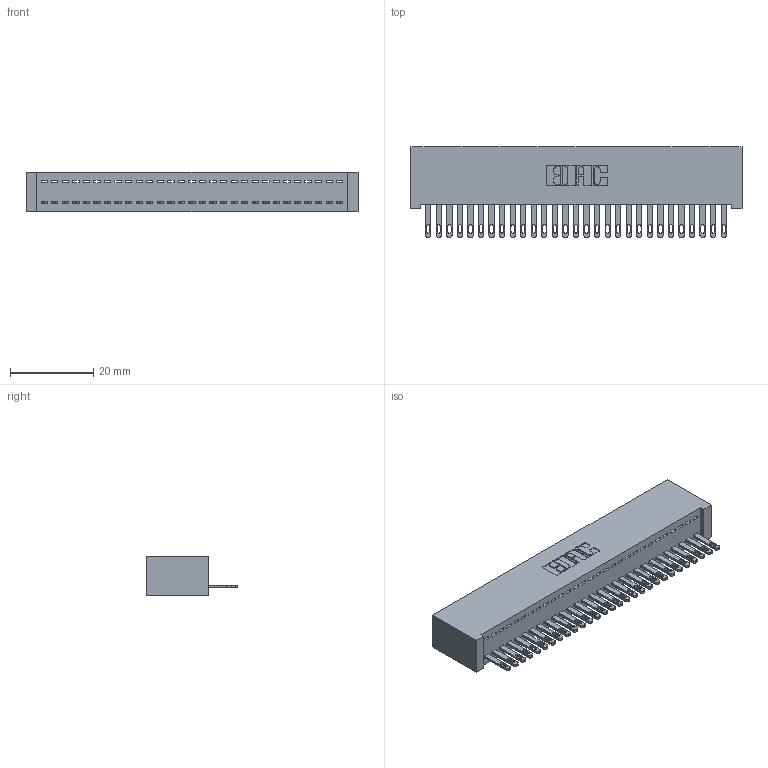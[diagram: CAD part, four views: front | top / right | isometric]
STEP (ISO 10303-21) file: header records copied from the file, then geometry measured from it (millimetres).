
FILE_DESCRIPTION (( 'STEP AP203' ), '1' );
FILE_NAME ('892-029-500-101.STEP', '2020-09-21T14:58:40', ( '' ), ( '' ), 'SwSTEP 2.0', 'SolidWorks 2020', '' );
FILE_SCHEMA (( 'CONFIG_CONTROL_DESIGN' ));
Length unit declared in the file: inch
Products named in the file (3): 842 Part_Lugless; 892-029-500-101; 345-292-001_345-293-100
Assembly tree (30 placements, depth 2):
  892-029-500-101
    842 Part_Lugless
    345-292-001_345-293-100  x29
Bounding box: 79.91 x 21.85 x 9.4 mm (x, y, z)
Volume: 7385.4 mm3; surface area: 10982.8 mm2
Topology: 30 solids, 30 shells, 1668 faces, 5147 edges, 3430 vertices
Faces by surface type: plane 1106, cylinder 562
Entity records: 18931 total; most frequent: CARTESIAN_POINT 3273, ORIENTED_EDGE 3238, DIRECTION 2781, EDGE_CURVE 1619, LINE 1495, VECTOR 1495, VERTEX_POINT 1078, AXIS2_PLACEMENT_3D 643
